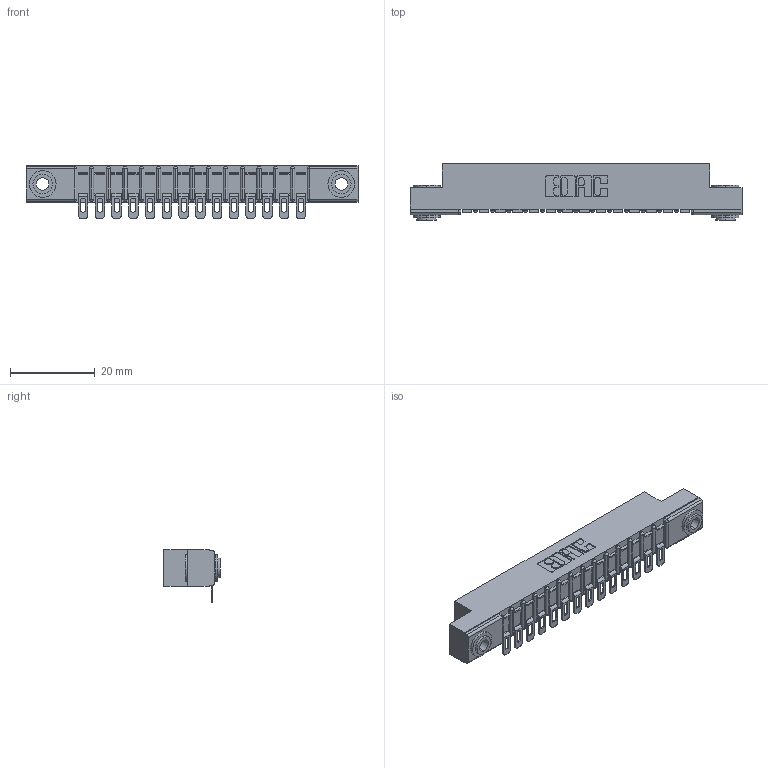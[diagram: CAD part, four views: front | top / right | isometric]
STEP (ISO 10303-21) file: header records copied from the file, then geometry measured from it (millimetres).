
FILE_DESCRIPTION (( 'STEP AP203' ), '1' );
FILE_NAME ('307-014-554-103.STEP', '2019-09-04T20:42:14', ( '' ), ( '' ), 'SwSTEP 2.0', 'SolidWorks 2016', '' );
FILE_SCHEMA (( 'CONFIG_CONTROL_DESIGN' ));
Length unit declared in the file: inch
Products named in the file (4): 307-290-002_554; 345-250-002_345-250-002-102; 307 Part_.156 Dia Mounting Holes; 307-014-554-103
Assembly tree (17 placements, depth 2):
  307-014-554-103
    307 Part_.156 Dia Mounting Holes
    307-290-002_554  x14
    345-250-002_345-250-002-102  x2
Bounding box: 78.49 x 13.36 x 12.52 mm (x, y, z)
Volume: 5183.7 mm3; surface area: 9284.9 mm2
Topology: 17 solids, 17 shells, 1319 faces, 3977 edges, 2606 vertices
Faces by surface type: plane 738, cylinder 543, sphere 30, cone 8
Entity records: 17484 total; most frequent: CARTESIAN_POINT 2923, ORIENTED_EDGE 2904, DIRECTION 2874, EDGE_CURVE 1452, VECTOR 1084, LINE 1084, VERTEX_POINT 944, AXIS2_PLACEMENT_3D 895
